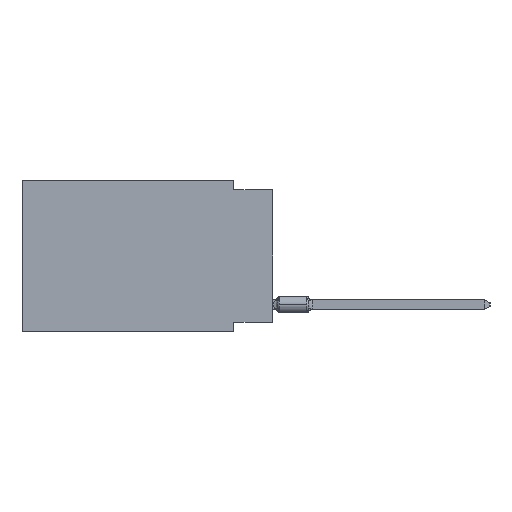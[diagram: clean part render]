
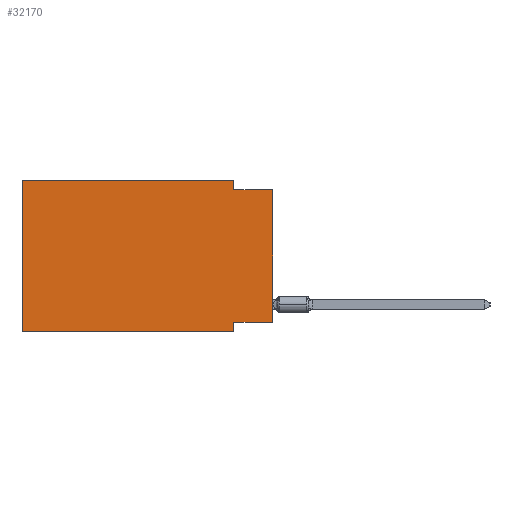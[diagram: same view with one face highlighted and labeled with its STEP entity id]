
A CAD part, left-side view. The second image highlights one B-rep face of the part: STEP entity #32170.
In plain terms, the highlighted planar face has unit normal (-1, 0, 0).
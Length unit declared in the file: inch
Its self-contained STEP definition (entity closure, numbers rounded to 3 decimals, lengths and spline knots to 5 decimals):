
#1325 = FACE_OUTER_BOUND ( 'NONE', #16913, .T. ) ;
#1380 = CARTESIAN_POINT ( 'NONE',  ( 0., 0., -0.025 ) ) ;
#1621 = VERTEX_POINT ( 'NONE', #11464 ) ;
#2596 = ORIENTED_EDGE ( 'NONE', *, *, #5619, .T. ) ;
#3602 = CARTESIAN_POINT ( 'NONE',  ( 0., 0.1, 0. ) ) ;
#3967 = LINE ( 'NONE', #4466, #16965 ) ;
#4466 = CARTESIAN_POINT ( 'NONE',  ( 0., 0.645, -0.39 ) ) ;
#4718 = VECTOR ( 'NONE', #18177, 39.37008 ) ;
#5010 = DIRECTION ( 'NONE',  ( 0., 0., 1. ) ) ;
#5355 = LINE ( 'NONE', #23061, #4718 ) ;
#5619 = EDGE_CURVE ( 'NONE', #17666, #6518, #3967, .T. ) ;
#5874 = CARTESIAN_POINT ( 'NONE',  ( 0., 0., 0. ) ) ;
#6518 = VERTEX_POINT ( 'NONE', #13838 ) ;
#7026 = CARTESIAN_POINT ( 'NONE',  ( 0., 0.645, -0.39 ) ) ;
#7808 = VECTOR ( 'NONE', #16151, 39.37008 ) ;
#8488 = DIRECTION ( 'NONE',  ( 0., 0., -1. ) ) ;
#9078 = LINE ( 'NONE', #5874, #7808 ) ;
#11170 = LINE ( 'NONE', #3602, #31559 ) ;
#11464 = CARTESIAN_POINT ( 'NONE',  ( 0., 0.1, -0.365 ) ) ;
#11545 = ORIENTED_EDGE ( 'NONE', *, *, #24497, .F. ) ;
#11602 = PLANE ( 'NONE',  #33078 ) ;
#12907 = CARTESIAN_POINT ( 'NONE',  ( 0., 0., -0.025 ) ) ;
#13017 = VERTEX_POINT ( 'NONE', #18192 ) ;
#13149 = CARTESIAN_POINT ( 'NONE',  ( 0., 0.1, 0. ) ) ;
#13838 = CARTESIAN_POINT ( 'NONE',  ( 0., 0.1, -0.39 ) ) ;
#14009 = LINE ( 'NONE', #24291, #15234 ) ;
#14515 = CARTESIAN_POINT ( 'NONE',  ( 0., 0., -0.365 ) ) ;
#15104 = DIRECTION ( 'NONE',  ( 0., -1., 0. ) ) ;
#15234 = VECTOR ( 'NONE', #21758, 39.37008 ) ;
#15722 = VECTOR ( 'NONE', #15104, 39.37008 ) ;
#16151 = DIRECTION ( 'NONE',  ( 0., 0., 1. ) ) ;
#16761 = CARTESIAN_POINT ( 'NONE',  ( 0., 0.1, -0.39 ) ) ;
#16913 = EDGE_LOOP ( 'NONE', ( #30815, #29461, #27649, #25677, #11545, #2596, #28574, #20843 ) ) ;
#16965 = VECTOR ( 'NONE', #27407, 39.37008 ) ;
#17589 = CARTESIAN_POINT ( 'NONE',  ( 0., 0.1, -0.025 ) ) ;
#17666 = VERTEX_POINT ( 'NONE', #7026 ) ;
#18177 = DIRECTION ( 'NONE',  ( 0., 1., 0. ) ) ;
#18192 = CARTESIAN_POINT ( 'NONE',  ( 0., 0.645, 0. ) ) ;
#19546 = DIRECTION ( 'NONE',  ( 1., 0., 0. ) ) ;
#20194 = VECTOR ( 'NONE', #22750, 39.37008 ) ;
#20356 = VERTEX_POINT ( 'NONE', #1380 ) ;
#20645 = VERTEX_POINT ( 'NONE', #13149 ) ;
#20843 = ORIENTED_EDGE ( 'NONE', *, *, #28679, .F. ) ;
#20879 = EDGE_CURVE ( 'NONE', #26687, #20356, #30640, .T. ) ;
#21553 = CARTESIAN_POINT ( 'NONE',  ( 0., 0.645, 0. ) ) ;
#21758 = DIRECTION ( 'NONE',  ( 0., -1., 0. ) ) ;
#22750 = DIRECTION ( 'NONE',  ( 0., 0., -1. ) ) ;
#23061 = CARTESIAN_POINT ( 'NONE',  ( 0., 0., -0.365 ) ) ;
#23933 = EDGE_CURVE ( 'NONE', #1621, #6518, #29759, .T. ) ;
#24239 = EDGE_CURVE ( 'NONE', #30621, #20356, #9078, .T. ) ;
#24291 = CARTESIAN_POINT ( 'NONE',  ( 0., 0.645, 0. ) ) ;
#24497 = EDGE_CURVE ( 'NONE', #17666, #13017, #25418, .T. ) ;
#25418 = LINE ( 'NONE', #28119, #32624 ) ;
#25677 = ORIENTED_EDGE ( 'NONE', *, *, #30517, .F. ) ;
#26518 = EDGE_CURVE ( 'NONE', #20645, #26687, #11170, .T. ) ;
#26687 = VERTEX_POINT ( 'NONE', #17589 ) ;
#27407 = DIRECTION ( 'NONE',  ( 0., -1., 0. ) ) ;
#27649 = ORIENTED_EDGE ( 'NONE', *, *, #26518, .F. ) ;
#28119 = CARTESIAN_POINT ( 'NONE',  ( 0., 0.645, 0. ) ) ;
#28574 = ORIENTED_EDGE ( 'NONE', *, *, #23933, .F. ) ;
#28679 = EDGE_CURVE ( 'NONE', #30621, #1621, #5355, .T. ) ;
#29461 = ORIENTED_EDGE ( 'NONE', *, *, #20879, .F. ) ;
#29759 = LINE ( 'NONE', #16761, #20194 ) ;
#30517 = EDGE_CURVE ( 'NONE', #13017, #20645, #14009, .T. ) ;
#30621 = VERTEX_POINT ( 'NONE', #14515 ) ;
#30640 = LINE ( 'NONE', #12907, #15722 ) ;
#30815 = ORIENTED_EDGE ( 'NONE', *, *, #24239, .T. ) ;
#31559 = VECTOR ( 'NONE', #8488, 39.37008 ) ;
#32170 = ADVANCED_FACE ( 'NONE', ( #1325 ), #11602, .F. ) ;
#32356 = DIRECTION ( 'NONE',  ( 0., 0., -1. ) ) ;
#32624 = VECTOR ( 'NONE', #5010, 39.37008 ) ;
#33078 = AXIS2_PLACEMENT_3D ( 'NONE', #21553, #19546, #32356 ) ;
